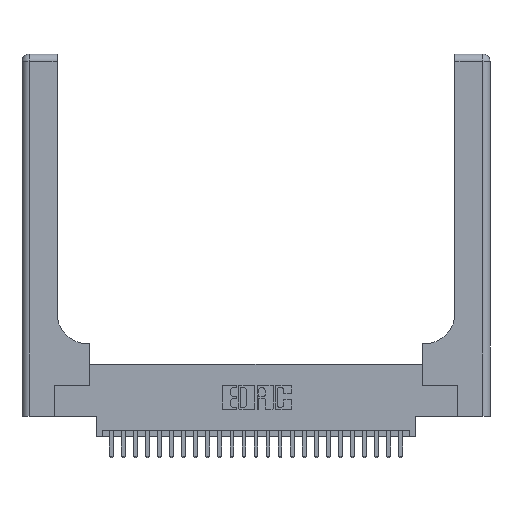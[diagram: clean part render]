
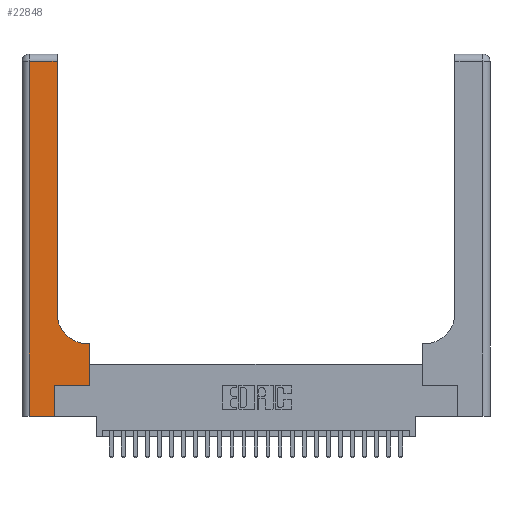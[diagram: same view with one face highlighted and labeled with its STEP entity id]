
A CAD part, top view. The second image highlights one B-rep face of the part: STEP entity #22848.
In plain terms, the highlighted planar face has unit normal (0, 0, 1).
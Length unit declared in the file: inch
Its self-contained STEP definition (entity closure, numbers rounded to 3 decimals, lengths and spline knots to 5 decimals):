
#40 = LINE ( 'NONE', #13480, #5799 ) ;
#57 = EDGE_CURVE ( 'NONE', #7436, #14977, #9359, .T. ) ;
#234 = VERTEX_POINT ( 'NONE', #13594 ) ;
#679 = VERTEX_POINT ( 'NONE', #10525 ) ;
#720 = CARTESIAN_POINT ( 'NONE',  ( 0.2915, 3., 0.37 ) ) ;
#775 = LINE ( 'NONE', #7994, #12086 ) ;
#999 = DIRECTION ( 'NONE',  ( 0., 1., 0. ) ) ;
#1447 = CARTESIAN_POINT ( 'NONE',  ( 0.269, 0.25, 0.37 ) ) ;
#2477 = CARTESIAN_POINT ( 'NONE',  ( 0., 0., 0.37 ) ) ;
#3060 = EDGE_CURVE ( 'NONE', #4236, #25438, #4894, .T. ) ;
#3065 = VECTOR ( 'NONE', #999, 39.37008 ) ;
#3190 = CARTESIAN_POINT ( 'NONE',  ( 0., 3., 0.37 ) ) ;
#4137 = CARTESIAN_POINT ( 'NONE',  ( 0.269, 0., 0.37 ) ) ;
#4236 = VERTEX_POINT ( 'NONE', #13192 ) ;
#4894 = LINE ( 'NONE', #4137, #10499 ) ;
#4964 = LINE ( 'NONE', #2477, #15516 ) ;
#5150 = ORIENTED_EDGE ( 'NONE', *, *, #23969, .T. ) ;
#5326 = DIRECTION ( 'NONE',  ( -1., 0., 0. ) ) ;
#5704 = VECTOR ( 'NONE', #9944, 39.37008 ) ;
#5799 = VECTOR ( 'NONE', #7145, 39.37008 ) ;
#6072 = ORIENTED_EDGE ( 'NONE', *, *, #26895, .T. ) ;
#7145 = DIRECTION ( 'NONE',  ( 0., -1., 0. ) ) ;
#7436 = VERTEX_POINT ( 'NONE', #20470 ) ;
#7452 = CARTESIAN_POINT ( 'NONE',  ( 0.5585, 0.25, 0.37 ) ) ;
#7994 = CARTESIAN_POINT ( 'NONE',  ( 0.2915, 0.6, 0.37 ) ) ;
#8998 = VECTOR ( 'NONE', #20006, 39.37008 ) ;
#9201 = ORIENTED_EDGE ( 'NONE', *, *, #21308, .T. ) ;
#9359 = LINE ( 'NONE', #720, #3065 ) ;
#9944 = DIRECTION ( 'NONE',  ( -1., 0., 0. ) ) ;
#10285 = EDGE_CURVE ( 'NONE', #679, #234, #775, .T. ) ;
#10369 = DIRECTION ( 'NONE',  ( 1., 0., 0. ) ) ;
#10499 = VECTOR ( 'NONE', #16746, 39.37008 ) ;
#10525 = CARTESIAN_POINT ( 'NONE',  ( 0.5585, 0.6, 0.37 ) ) ;
#10753 = AXIS2_PLACEMENT_3D ( 'NONE', #11233, #25907, #13343 ) ;
#11233 = CARTESIAN_POINT ( 'NONE',  ( 0.5415, 0.85, 0.37 ) ) ;
#11319 = LINE ( 'NONE', #26625, #5704 ) ;
#12030 = CARTESIAN_POINT ( 'NONE',  ( 0.06, 2.94, 0.37 ) ) ;
#12086 = VECTOR ( 'NONE', #22692, 39.37008 ) ;
#12554 = LINE ( 'NONE', #20823, #17486 ) ;
#12618 = VERTEX_POINT ( 'NONE', #18478 ) ;
#13113 = DIRECTION ( 'NONE',  ( 1., 0., 0. ) ) ;
#13192 = CARTESIAN_POINT ( 'NONE',  ( 0.269, 0., 0.37 ) ) ;
#13343 = DIRECTION ( 'NONE',  ( 1., 0., 0. ) ) ;
#13435 = VERTEX_POINT ( 'NONE', #13481 ) ;
#13480 = CARTESIAN_POINT ( 'NONE',  ( 0.06, 3., 0.37 ) ) ;
#13481 = CARTESIAN_POINT ( 'NONE',  ( 0.06, 0., 0.37 ) ) ;
#13594 = CARTESIAN_POINT ( 'NONE',  ( 0.5415, 0.6, 0.37 ) ) ;
#13706 = PLANE ( 'NONE',  #24839 ) ;
#14307 = ORIENTED_EDGE ( 'NONE', *, *, #10285, .T. ) ;
#14977 = VERTEX_POINT ( 'NONE', #22571 ) ;
#15516 = VECTOR ( 'NONE', #13113, 39.37008 ) ;
#16746 = DIRECTION ( 'NONE',  ( 0., 1., 0. ) ) ;
#17003 = ORIENTED_EDGE ( 'NONE', *, *, #57, .T. ) ;
#17486 = VECTOR ( 'NONE', #10369, 39.37008 ) ;
#17922 = DIRECTION ( 'NONE',  ( 0., 0., -1. ) ) ;
#18436 = ORIENTED_EDGE ( 'NONE', *, *, #22855, .T. ) ;
#18478 = CARTESIAN_POINT ( 'NONE',  ( 0.5585, 0.25, 0.37 ) ) ;
#19742 = VERTEX_POINT ( 'NONE', #12030 ) ;
#20006 = DIRECTION ( 'NONE',  ( 0., 1., 0. ) ) ;
#20055 = ORIENTED_EDGE ( 'NONE', *, *, #22745, .T. ) ;
#20470 = CARTESIAN_POINT ( 'NONE',  ( 0.2915, 0.85, 0.37 ) ) ;
#20823 = CARTESIAN_POINT ( 'NONE',  ( 0.269, 0.25, 0.37 ) ) ;
#21308 = EDGE_CURVE ( 'NONE', #25438, #12618, #12554, .T. ) ;
#21929 = EDGE_LOOP ( 'NONE', ( #17003, #26809, #6072, #5150, #22355, #9201, #18436, #14307, #20055 ) ) ;
#22132 = CIRCLE ( 'NONE', #10753, 0.25 ) ;
#22355 = ORIENTED_EDGE ( 'NONE', *, *, #3060, .T. ) ;
#22485 = EDGE_CURVE ( 'NONE', #14977, #19742, #11319, .T. ) ;
#22571 = CARTESIAN_POINT ( 'NONE',  ( 0.2915, 2.94, 0.37 ) ) ;
#22692 = DIRECTION ( 'NONE',  ( -1., 0., 0. ) ) ;
#22745 = EDGE_CURVE ( 'NONE', #234, #7436, #22132, .T. ) ;
#22848 = ADVANCED_FACE ( 'NONE', ( #25741 ), #13706, .F. ) ;
#22855 = EDGE_CURVE ( 'NONE', #12618, #679, #26370, .T. ) ;
#23969 = EDGE_CURVE ( 'NONE', #13435, #4236, #4964, .T. ) ;
#24839 = AXIS2_PLACEMENT_3D ( 'NONE', #3190, #17922, #5326 ) ;
#25438 = VERTEX_POINT ( 'NONE', #1447 ) ;
#25741 = FACE_OUTER_BOUND ( 'NONE', #21929, .T. ) ;
#25907 = DIRECTION ( 'NONE',  ( 0., 0., -1. ) ) ;
#26370 = LINE ( 'NONE', #7452, #8998 ) ;
#26625 = CARTESIAN_POINT ( 'NONE',  ( 0., 2.94, 0.37 ) ) ;
#26809 = ORIENTED_EDGE ( 'NONE', *, *, #22485, .T. ) ;
#26895 = EDGE_CURVE ( 'NONE', #19742, #13435, #40, .T. ) ;
